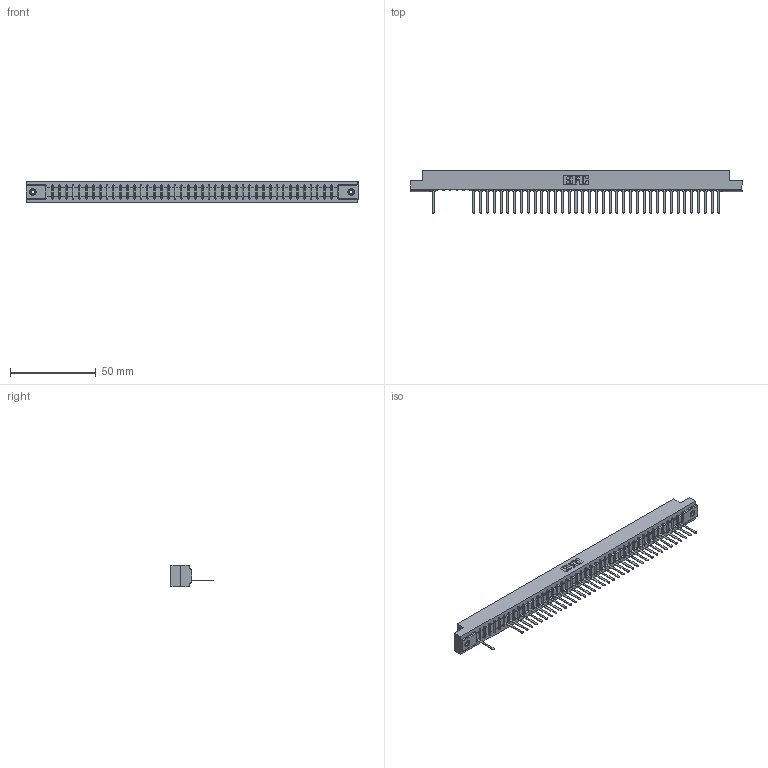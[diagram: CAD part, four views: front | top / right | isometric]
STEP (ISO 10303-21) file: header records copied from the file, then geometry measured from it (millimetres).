
FILE_DESCRIPTION (( 'STEP AP203' ), '1' );
FILE_NAME ('357-043-541-108.STEP', '2018-08-11T10:20:11', ( '' ), ( '' ), 'SwSTEP 2.0', 'SolidWorks 2016', '' );
FILE_SCHEMA (( 'CONFIG_CONTROL_DESIGN' ));
Length unit declared in the file: inch
Products named in the file (4): 307-290-002_541; 345-250-001_345-250-003-102; 357-043-541-108; 307 Part_.156 Dia Mounting Holes
Assembly tree (41 placements, depth 2):
  357-043-541-108
    307 Part_.156 Dia Mounting Holes
    307-290-002_541  x38
    345-250-001_345-250-003-102  x2
Bounding box: 193.4 x 24.59 x 12.7 mm (x, y, z)
Volume: 20659.3 mm3; surface area: 25780.9 mm2
Topology: 41 solids, 41 shells, 3134 faces, 9595 edges, 6270 vertices
Faces by surface type: plane 1872, cylinder 1158, sphere 88, cone 12, torus 4
Entity records: 38483 total; most frequent: CARTESIAN_POINT 6494, ORIENTED_EDGE 6482, DIRECTION 6313, EDGE_CURVE 3241, LINE 2483, VECTOR 2483, VERTEX_POINT 2096, AXIS2_PLACEMENT_3D 1915
